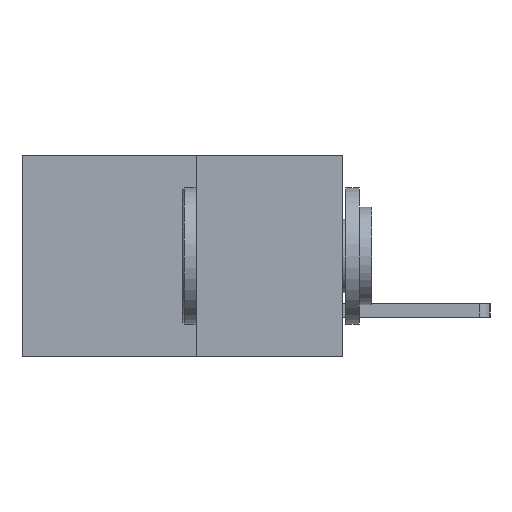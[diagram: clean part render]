
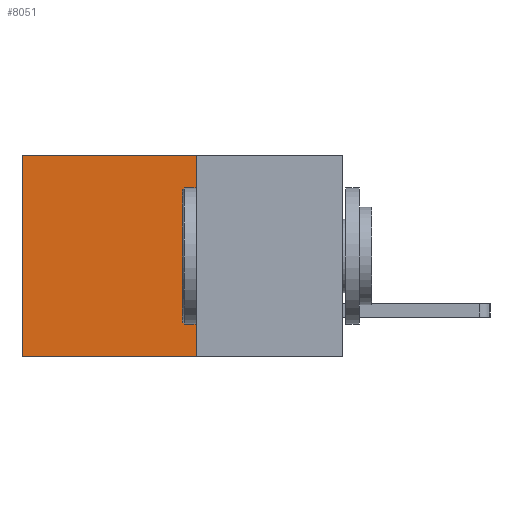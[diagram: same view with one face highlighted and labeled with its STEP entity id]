
A CAD part, left-side view. The second image highlights one B-rep face of the part: STEP entity #8051.
In plain terms, the highlighted planar face has unit normal (-1, 0, 0).
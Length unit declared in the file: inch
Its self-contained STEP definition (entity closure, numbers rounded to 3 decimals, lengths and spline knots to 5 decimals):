
#137 = EDGE_CURVE ( 'NONE', #8013, #9487, #2079, .T. ) ;
#401 = CARTESIAN_POINT ( 'NONE',  ( 0.277, 0.59, -0.37 ) ) ;
#622 = VERTEX_POINT ( 'NONE', #9288 ) ;
#876 = VERTEX_POINT ( 'NONE', #2444 ) ;
#1135 = CARTESIAN_POINT ( 'NONE',  ( 0.277, 0.27, 0. ) ) ;
#1193 = VECTOR ( 'NONE', #5899, 39.37008 ) ;
#1384 = DIRECTION ( 'NONE',  ( 0., 0., -1. ) ) ;
#1852 = EDGE_CURVE ( 'NONE', #622, #9487, #9210, .T. ) ;
#1871 = CARTESIAN_POINT ( 'NONE',  ( 0.277, 0.27, -0.37 ) ) ;
#2079 = LINE ( 'NONE', #6798, #3897 ) ;
#2444 = CARTESIAN_POINT ( 'NONE',  ( 0.277, 0.27, 0. ) ) ;
#2967 = LINE ( 'NONE', #1135, #8672 ) ;
#3897 = VECTOR ( 'NONE', #8824, 39.37008 ) ;
#4543 = ORIENTED_EDGE ( 'NONE', *, *, #1852, .F. ) ;
#4590 = EDGE_CURVE ( 'NONE', #876, #622, #8340, .T. ) ;
#5166 = EDGE_CURVE ( 'NONE', #876, #8013, #2967, .T. ) ;
#5899 = DIRECTION ( 'NONE',  ( 0., 1., 0. ) ) ;
#6021 = ORIENTED_EDGE ( 'NONE', *, *, #137, .T. ) ;
#6209 = VECTOR ( 'NONE', #1384, 39.37008 ) ;
#6256 = DIRECTION ( 'NONE',  ( 0., 1., 0. ) ) ;
#6643 = AXIS2_PLACEMENT_3D ( 'NONE', #8879, #8763, #8754 ) ;
#6798 = CARTESIAN_POINT ( 'NONE',  ( 0.277, 0.59, -0.37 ) ) ;
#7035 = ORIENTED_EDGE ( 'NONE', *, *, #4590, .F. ) ;
#7227 = CARTESIAN_POINT ( 'NONE',  ( 0.277, 0.27, -0.37 ) ) ;
#8013 = VERTEX_POINT ( 'NONE', #9121 ) ;
#8051 = ADVANCED_FACE ( 'NONE', ( #8390 ), #8768, .F. ) ;
#8340 = LINE ( 'NONE', #1871, #6209 ) ;
#8361 = EDGE_LOOP ( 'NONE', ( #6021, #4543, #7035, #9408 ) ) ;
#8390 = FACE_OUTER_BOUND ( 'NONE', #8361, .T. ) ;
#8672 = VECTOR ( 'NONE', #6256, 39.37008 ) ;
#8754 = DIRECTION ( 'NONE',  ( 0., 0., -1. ) ) ;
#8763 = DIRECTION ( 'NONE',  ( 1., 0., 0. ) ) ;
#8768 = PLANE ( 'NONE',  #6643 ) ;
#8824 = DIRECTION ( 'NONE',  ( 0., 0., -1. ) ) ;
#8879 = CARTESIAN_POINT ( 'NONE',  ( 0.277, 0.27, -0.37 ) ) ;
#9121 = CARTESIAN_POINT ( 'NONE',  ( 0.277, 0.59, 0. ) ) ;
#9210 = LINE ( 'NONE', #7227, #1193 ) ;
#9288 = CARTESIAN_POINT ( 'NONE',  ( 0.277, 0.27, -0.37 ) ) ;
#9408 = ORIENTED_EDGE ( 'NONE', *, *, #5166, .T. ) ;
#9487 = VERTEX_POINT ( 'NONE', #401 ) ;
